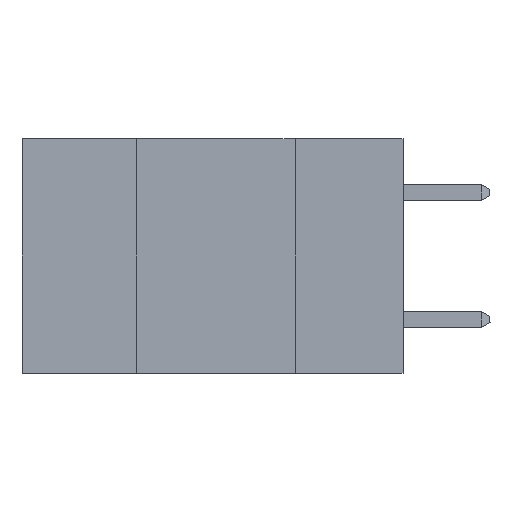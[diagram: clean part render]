
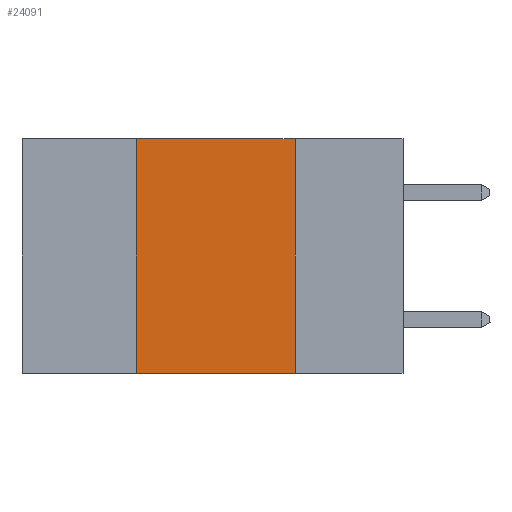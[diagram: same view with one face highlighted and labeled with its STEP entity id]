
A CAD part, left-side view. The second image highlights one B-rep face of the part: STEP entity #24091.
In plain terms, the highlighted planar face has unit normal (-1, 0, 0).
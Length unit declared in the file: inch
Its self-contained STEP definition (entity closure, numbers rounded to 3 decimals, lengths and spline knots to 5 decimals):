
#731 = CARTESIAN_POINT ( 'NONE',  ( 0., 0.42, 0. ) ) ;
#1999 = VECTOR ( 'NONE', #3839, 39.37008 ) ;
#2802 = VERTEX_POINT ( 'NONE', #31231 ) ;
#3307 = DIRECTION ( 'NONE',  ( 0., 0., -1. ) ) ;
#3839 = DIRECTION ( 'NONE',  ( 0., 0., 1. ) ) ;
#4403 = EDGE_CURVE ( 'NONE', #10293, #16067, #28639, .T. ) ;
#5794 = DIRECTION ( 'NONE',  ( 0., -1., 0. ) ) ;
#6628 = CARTESIAN_POINT ( 'NONE',  ( 0., 0.42, 0. ) ) ;
#6804 = ORIENTED_EDGE ( 'NONE', *, *, #23853, .T. ) ;
#10293 = VERTEX_POINT ( 'NONE', #23837 ) ;
#11356 = LINE ( 'NONE', #18709, #14329 ) ;
#11761 = DIRECTION ( 'NONE',  ( 0., 0., -1. ) ) ;
#13104 = PLANE ( 'NONE',  #23208 ) ;
#13501 = VECTOR ( 'NONE', #11761, 39.37008 ) ;
#14211 = LINE ( 'NONE', #24158, #13501 ) ;
#14329 = VECTOR ( 'NONE', #18532, 39.37008 ) ;
#15456 = CARTESIAN_POINT ( 'NONE',  ( 0., 0.6, 0. ) ) ;
#15727 = FACE_OUTER_BOUND ( 'NONE', #22430, .T. ) ;
#16067 = VERTEX_POINT ( 'NONE', #731 ) ;
#16455 = EDGE_CURVE ( 'NONE', #16067, #2802, #28145, .T. ) ;
#18021 = CARTESIAN_POINT ( 'NONE',  ( 0., 0.6, 0. ) ) ;
#18532 = DIRECTION ( 'NONE',  ( 0., -1., 0. ) ) ;
#18617 = ORIENTED_EDGE ( 'NONE', *, *, #16455, .F. ) ;
#18709 = CARTESIAN_POINT ( 'NONE',  ( 0., 0.6, -0.37 ) ) ;
#19833 = VERTEX_POINT ( 'NONE', #23935 ) ;
#22430 = EDGE_LOOP ( 'NONE', ( #29628, #18617, #32073, #6804 ) ) ;
#23208 = AXIS2_PLACEMENT_3D ( 'NONE', #18021, #25640, #3307 ) ;
#23837 = CARTESIAN_POINT ( 'NONE',  ( 0., 0.42, -0.37 ) ) ;
#23853 = EDGE_CURVE ( 'NONE', #10293, #19833, #11356, .T. ) ;
#23935 = CARTESIAN_POINT ( 'NONE',  ( 0., 0.17, -0.37 ) ) ;
#24091 = ADVANCED_FACE ( 'NONE', ( #15727 ), #13104, .F. ) ;
#24158 = CARTESIAN_POINT ( 'NONE',  ( 0., 0.17, 0. ) ) ;
#24921 = VECTOR ( 'NONE', #5794, 39.37008 ) ;
#25640 = DIRECTION ( 'NONE',  ( 1., 0., 0. ) ) ;
#28145 = LINE ( 'NONE', #15456, #24921 ) ;
#28639 = LINE ( 'NONE', #6628, #1999 ) ;
#29628 = ORIENTED_EDGE ( 'NONE', *, *, #30567, .F. ) ;
#30567 = EDGE_CURVE ( 'NONE', #2802, #19833, #14211, .T. ) ;
#31231 = CARTESIAN_POINT ( 'NONE',  ( 0., 0.17, 0. ) ) ;
#32073 = ORIENTED_EDGE ( 'NONE', *, *, #4403, .F. ) ;
